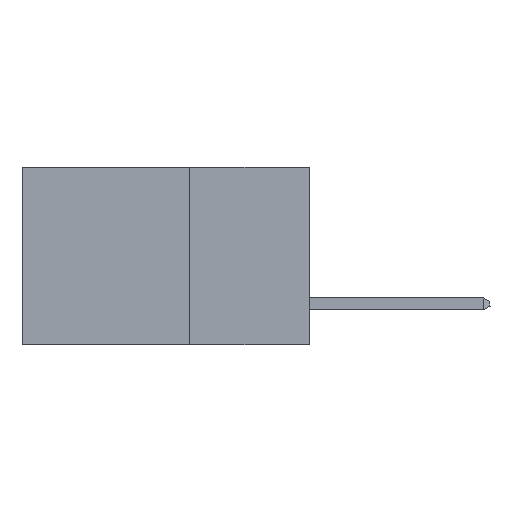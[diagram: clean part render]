
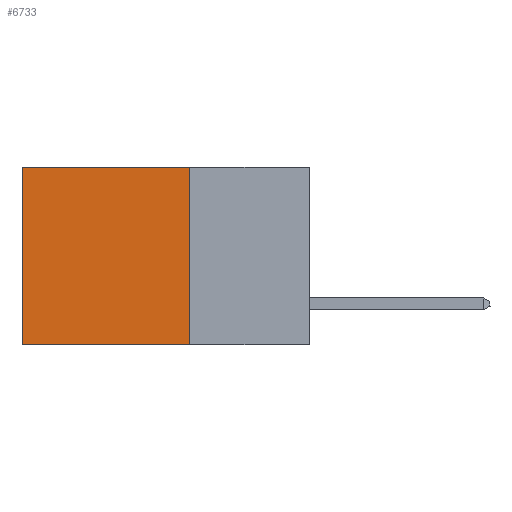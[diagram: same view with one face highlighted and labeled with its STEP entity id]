
A CAD part, left-side view. The second image highlights one B-rep face of the part: STEP entity #6733.
In plain terms, the highlighted planar face has unit normal (-1, 0, 0).
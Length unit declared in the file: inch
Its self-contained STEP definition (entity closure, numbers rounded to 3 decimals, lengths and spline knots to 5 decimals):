
#552 = DIRECTION ( 'NONE',  ( 0., 0., -1. ) ) ;
#821 = FACE_OUTER_BOUND ( 'NONE', #11584, .T. ) ;
#1593 = VERTEX_POINT ( 'NONE', #7836 ) ;
#1970 = DIRECTION ( 'NONE',  ( 0., 0., -1. ) ) ;
#2155 = VERTEX_POINT ( 'NONE', #6371 ) ;
#2206 = ORIENTED_EDGE ( 'NONE', *, *, #10433, .T. ) ;
#3145 = LINE ( 'NONE', #12740, #11091 ) ;
#4161 = CARTESIAN_POINT ( 'NONE',  ( 0.2875, 0.6, -0.37 ) ) ;
#4476 = LINE ( 'NONE', #5866, #7050 ) ;
#4724 = EDGE_CURVE ( 'NONE', #8568, #1593, #5007, .T. ) ;
#4921 = DIRECTION ( 'NONE',  ( 1., 0., 0. ) ) ;
#5007 = LINE ( 'NONE', #11379, #7617 ) ;
#5025 = EDGE_CURVE ( 'NONE', #8568, #2155, #3145, .T. ) ;
#5071 = ORIENTED_EDGE ( 'NONE', *, *, #11993, .F. ) ;
#5866 = CARTESIAN_POINT ( 'NONE',  ( 0.2875, 0.25, -0.37 ) ) ;
#6247 = ORIENTED_EDGE ( 'NONE', *, *, #5025, .F. ) ;
#6371 = CARTESIAN_POINT ( 'NONE',  ( 0.2875, 0.25, -0.37 ) ) ;
#6733 = ADVANCED_FACE ( 'NONE', ( #821 ), #11282, .F. ) ;
#7048 = CARTESIAN_POINT ( 'NONE',  ( 0.2875, 0.25, 0. ) ) ;
#7050 = VECTOR ( 'NONE', #9118, 39.37008 ) ;
#7617 = VECTOR ( 'NONE', #12498, 39.37008 ) ;
#7836 = CARTESIAN_POINT ( 'NONE',  ( 0.2875, 0.6, 0. ) ) ;
#8236 = DIRECTION ( 'NONE',  ( 0., 0., -1. ) ) ;
#8568 = VERTEX_POINT ( 'NONE', #7048 ) ;
#8591 = ORIENTED_EDGE ( 'NONE', *, *, #4724, .T. ) ;
#8667 = VECTOR ( 'NONE', #1970, 39.37008 ) ;
#9118 = DIRECTION ( 'NONE',  ( 0., 1., 0. ) ) ;
#10433 = EDGE_CURVE ( 'NONE', #1593, #12292, #12482, .T. ) ;
#11091 = VECTOR ( 'NONE', #8236, 39.37008 ) ;
#11140 = AXIS2_PLACEMENT_3D ( 'NONE', #12772, #4921, #552 ) ;
#11282 = PLANE ( 'NONE',  #11140 ) ;
#11379 = CARTESIAN_POINT ( 'NONE',  ( 0.2875, 0.25, 0. ) ) ;
#11584 = EDGE_LOOP ( 'NONE', ( #2206, #5071, #6247, #8591 ) ) ;
#11993 = EDGE_CURVE ( 'NONE', #2155, #12292, #4476, .T. ) ;
#12292 = VERTEX_POINT ( 'NONE', #4161 ) ;
#12482 = LINE ( 'NONE', #13811, #8667 ) ;
#12498 = DIRECTION ( 'NONE',  ( 0., 1., 0. ) ) ;
#12740 = CARTESIAN_POINT ( 'NONE',  ( 0.2875, 0.25, 0. ) ) ;
#12772 = CARTESIAN_POINT ( 'NONE',  ( 0.2875, 0.25, 0. ) ) ;
#13811 = CARTESIAN_POINT ( 'NONE',  ( 0.2875, 0.6, 0. ) ) ;
